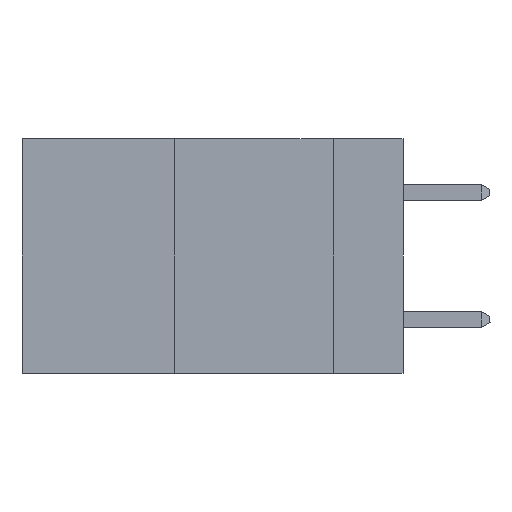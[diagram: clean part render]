
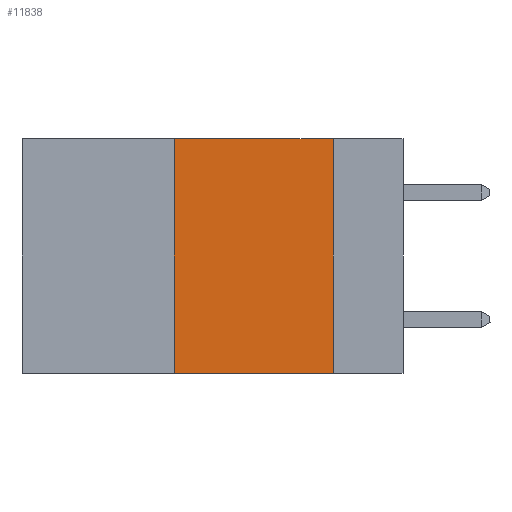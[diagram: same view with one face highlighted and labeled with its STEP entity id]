
A CAD part, left-side view. The second image highlights one B-rep face of the part: STEP entity #11838.
In plain terms, the highlighted planar face has unit normal (-1, 0, 0).
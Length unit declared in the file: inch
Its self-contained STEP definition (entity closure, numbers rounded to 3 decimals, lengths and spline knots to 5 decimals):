
#439 = CARTESIAN_POINT ( 'NONE',  ( 0., 0.36, 0. ) ) ;
#1072 = CARTESIAN_POINT ( 'NONE',  ( 0., 0.11, 0. ) ) ;
#1137 = LINE ( 'NONE', #12728, #6222 ) ;
#2082 = AXIS2_PLACEMENT_3D ( 'NONE', #7989, #9969, #4022 ) ;
#2084 = DIRECTION ( 'NONE',  ( 0., 0., -1. ) ) ;
#2582 = LINE ( 'NONE', #10184, #7943 ) ;
#2774 = EDGE_CURVE ( 'NONE', #10224, #6343, #12258, .T. ) ;
#4022 = DIRECTION ( 'NONE',  ( 0., 0., -1. ) ) ;
#4520 = VECTOR ( 'NONE', #2084, 39.37008 ) ;
#4773 = CARTESIAN_POINT ( 'NONE',  ( 0., 0.36, -0.37 ) ) ;
#6183 = CARTESIAN_POINT ( 'NONE',  ( 0., 0.6, -0.37 ) ) ;
#6222 = VECTOR ( 'NONE', #9855, 39.37008 ) ;
#6245 = ORIENTED_EDGE ( 'NONE', *, *, #9218, .F. ) ;
#6343 = VERTEX_POINT ( 'NONE', #6563 ) ;
#6460 = DIRECTION ( 'NONE',  ( 0., -1., 0. ) ) ;
#6563 = CARTESIAN_POINT ( 'NONE',  ( 0., 0.11, -0.37 ) ) ;
#7187 = DIRECTION ( 'NONE',  ( 0., -1., 0. ) ) ;
#7338 = VECTOR ( 'NONE', #6460, 39.37008 ) ;
#7440 = ORIENTED_EDGE ( 'NONE', *, *, #11118, .F. ) ;
#7451 = ORIENTED_EDGE ( 'NONE', *, *, #2774, .T. ) ;
#7574 = ORIENTED_EDGE ( 'NONE', *, *, #10628, .F. ) ;
#7943 = VECTOR ( 'NONE', #7187, 39.37008 ) ;
#7989 = CARTESIAN_POINT ( 'NONE',  ( 0., 0.6, 0. ) ) ;
#8179 = VERTEX_POINT ( 'NONE', #439 ) ;
#8485 = EDGE_LOOP ( 'NONE', ( #7574, #6245, #7440, #7451 ) ) ;
#9218 = EDGE_CURVE ( 'NONE', #8179, #10770, #2582, .T. ) ;
#9803 = LINE ( 'NONE', #1072, #4520 ) ;
#9855 = DIRECTION ( 'NONE',  ( 0., 0., 1. ) ) ;
#9969 = DIRECTION ( 'NONE',  ( 1., 0., 0. ) ) ;
#10184 = CARTESIAN_POINT ( 'NONE',  ( 0., 0.6, 0. ) ) ;
#10224 = VERTEX_POINT ( 'NONE', #4773 ) ;
#10628 = EDGE_CURVE ( 'NONE', #10770, #6343, #9803, .T. ) ;
#10770 = VERTEX_POINT ( 'NONE', #12287 ) ;
#11118 = EDGE_CURVE ( 'NONE', #10224, #8179, #1137, .T. ) ;
#11838 = ADVANCED_FACE ( 'NONE', ( #12649 ), #12832, .F. ) ;
#12258 = LINE ( 'NONE', #6183, #7338 ) ;
#12287 = CARTESIAN_POINT ( 'NONE',  ( 0., 0.11, 0. ) ) ;
#12649 = FACE_OUTER_BOUND ( 'NONE', #8485, .T. ) ;
#12728 = CARTESIAN_POINT ( 'NONE',  ( 0., 0.36, 0. ) ) ;
#12832 = PLANE ( 'NONE',  #2082 ) ;
